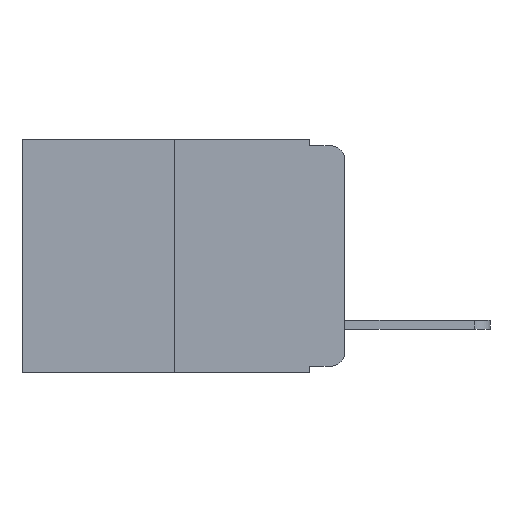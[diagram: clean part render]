
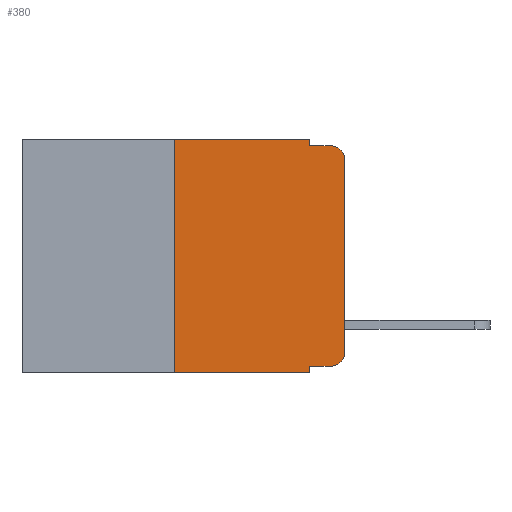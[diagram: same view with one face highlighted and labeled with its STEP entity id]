
A CAD part, left-side view. The second image highlights one B-rep face of the part: STEP entity #380.
In plain terms, the highlighted planar face has unit normal (-1, 0, 0).
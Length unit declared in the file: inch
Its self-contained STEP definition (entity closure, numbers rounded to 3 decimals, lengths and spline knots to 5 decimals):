
#11 = CARTESIAN_POINT ( 'NONE',  ( 0., 0.051, -0.333 ) ) ;
#145 = CARTESIAN_POINT ( 'NONE',  ( 0., 0., -0.03 ) ) ;
#380 = ADVANCED_FACE ( 'NONE', ( #26238 ), #19855, .F. ) ;
#389 = DIRECTION ( 'NONE',  ( 0., -1., 0. ) ) ;
#638 = VERTEX_POINT ( 'NONE', #8819 ) ;
#847 = DIRECTION ( 'NONE',  ( 0., 0., -1. ) ) ;
#1502 = LINE ( 'NONE', #21093, #23207 ) ;
#1549 = EDGE_CURVE ( 'NONE', #16674, #19604, #25883, .T. ) ;
#2672 = CARTESIAN_POINT ( 'NONE',  ( 0., 0.051, -0.333 ) ) ;
#2821 = DIRECTION ( 'NONE',  ( 1., 0., 0. ) ) ;
#3396 = ORIENTED_EDGE ( 'NONE', *, *, #11394, .F. ) ;
#3558 = VERTEX_POINT ( 'NONE', #25759 ) ;
#4065 = DIRECTION ( 'NONE',  ( 0., 0., -1. ) ) ;
#4387 = CARTESIAN_POINT ( 'NONE',  ( 0., 0.051, 0. ) ) ;
#4966 = ORIENTED_EDGE ( 'NONE', *, *, #20659, .F. ) ;
#5170 = VECTOR ( 'NONE', #23710, 39.37008 ) ;
#5179 = CARTESIAN_POINT ( 'NONE',  ( 0., 0.02, -0.03 ) ) ;
#5400 = CARTESIAN_POINT ( 'NONE',  ( 0., 0.051, -0.01 ) ) ;
#5989 = EDGE_CURVE ( 'NONE', #12069, #20249, #1502, .T. ) ;
#6025 = ORIENTED_EDGE ( 'NONE', *, *, #10478, .T. ) ;
#6357 = LINE ( 'NONE', #5400, #10859 ) ;
#6811 = VECTOR ( 'NONE', #18965, 39.37008 ) ;
#7145 = EDGE_CURVE ( 'NONE', #23434, #12368, #23987, .T. ) ;
#7279 = CARTESIAN_POINT ( 'NONE',  ( 0., 0.051, 0. ) ) ;
#7576 = VERTEX_POINT ( 'NONE', #20404 ) ;
#7579 = DIRECTION ( 'NONE',  ( 0., 0., -1. ) ) ;
#8819 = CARTESIAN_POINT ( 'NONE',  ( 0., 0., -0.313 ) ) ;
#8915 = ORIENTED_EDGE ( 'NONE', *, *, #20207, .T. ) ;
#9317 = ORIENTED_EDGE ( 'NONE', *, *, #16823, .F. ) ;
#9925 = CARTESIAN_POINT ( 'NONE',  ( 0., 0.473, 0. ) ) ;
#10348 = AXIS2_PLACEMENT_3D ( 'NONE', #23333, #2821, #18518 ) ;
#10478 = EDGE_CURVE ( 'NONE', #638, #13058, #14177, .T. ) ;
#10859 = VECTOR ( 'NONE', #23642, 39.37008 ) ;
#10998 = EDGE_LOOP ( 'NONE', ( #6025, #8915, #18679, #19288, #3396, #4966, #12213, #9317, #21693, #17779 ) ) ;
#11394 = EDGE_CURVE ( 'NONE', #3558, #16674, #15629, .T. ) ;
#12069 = VERTEX_POINT ( 'NONE', #15549 ) ;
#12213 = ORIENTED_EDGE ( 'NONE', *, *, #5989, .T. ) ;
#12259 = CARTESIAN_POINT ( 'NONE',  ( 0., 0., 0. ) ) ;
#12368 = VERTEX_POINT ( 'NONE', #16538 ) ;
#12529 = LINE ( 'NONE', #26191, #6811 ) ;
#13058 = VERTEX_POINT ( 'NONE', #145 ) ;
#14065 = CARTESIAN_POINT ( 'NONE',  ( 0., 0.051, 0. ) ) ;
#14177 = LINE ( 'NONE', #12259, #15356 ) ;
#14287 = DIRECTION ( 'NONE',  ( 0., 0., 1. ) ) ;
#14401 = DIRECTION ( 'NONE',  ( -1., 0., 0. ) ) ;
#14963 = EDGE_CURVE ( 'NONE', #19604, #7576, #6357, .T. ) ;
#15356 = VECTOR ( 'NONE', #14287, 39.37008 ) ;
#15549 = CARTESIAN_POINT ( 'NONE',  ( 0., 0.25, -0.343 ) ) ;
#15629 = LINE ( 'NONE', #9925, #20220 ) ;
#16182 = AXIS2_PLACEMENT_3D ( 'NONE', #25723, #14401, #847 ) ;
#16419 = LINE ( 'NONE', #14065, #5170 ) ;
#16538 = CARTESIAN_POINT ( 'NONE',  ( 0., 0.02, -0.333 ) ) ;
#16674 = VERTEX_POINT ( 'NONE', #7279 ) ;
#16823 = EDGE_CURVE ( 'NONE', #23434, #20249, #16419, .T. ) ;
#17143 = CIRCLE ( 'NONE', #16182, 0.02 ) ;
#17779 = ORIENTED_EDGE ( 'NONE', *, *, #23666, .T. ) ;
#17806 = CARTESIAN_POINT ( 'NONE',  ( 0., 0.051, -0.343 ) ) ;
#18518 = DIRECTION ( 'NONE',  ( 0., 0., -1. ) ) ;
#18679 = ORIENTED_EDGE ( 'NONE', *, *, #14963, .F. ) ;
#18965 = DIRECTION ( 'NONE',  ( 0., 0., 1. ) ) ;
#19009 = VECTOR ( 'NONE', #389, 39.37008 ) ;
#19288 = ORIENTED_EDGE ( 'NONE', *, *, #1549, .F. ) ;
#19308 = CIRCLE ( 'NONE', #20060, 0.02 ) ;
#19604 = VERTEX_POINT ( 'NONE', #24099 ) ;
#19671 = DIRECTION ( 'NONE',  ( -1., 0., 0. ) ) ;
#19855 = PLANE ( 'NONE',  #10348 ) ;
#20060 = AXIS2_PLACEMENT_3D ( 'NONE', #5179, #19671, #7579 ) ;
#20207 = EDGE_CURVE ( 'NONE', #13058, #7576, #19308, .T. ) ;
#20220 = VECTOR ( 'NONE', #25337, 39.37008 ) ;
#20249 = VERTEX_POINT ( 'NONE', #17806 ) ;
#20404 = CARTESIAN_POINT ( 'NONE',  ( 0., 0.02, -0.01 ) ) ;
#20659 = EDGE_CURVE ( 'NONE', #12069, #3558, #12529, .T. ) ;
#21059 = DIRECTION ( 'NONE',  ( 0., -1., 0. ) ) ;
#21093 = CARTESIAN_POINT ( 'NONE',  ( 0., 0.473, -0.343 ) ) ;
#21693 = ORIENTED_EDGE ( 'NONE', *, *, #7145, .T. ) ;
#23207 = VECTOR ( 'NONE', #21059, 39.37008 ) ;
#23333 = CARTESIAN_POINT ( 'NONE',  ( 0., 0.473, 0. ) ) ;
#23434 = VERTEX_POINT ( 'NONE', #2672 ) ;
#23642 = DIRECTION ( 'NONE',  ( 0., -1., 0. ) ) ;
#23666 = EDGE_CURVE ( 'NONE', #12368, #638, #17143, .T. ) ;
#23710 = DIRECTION ( 'NONE',  ( 0., 0., -1. ) ) ;
#23987 = LINE ( 'NONE', #11, #19009 ) ;
#24099 = CARTESIAN_POINT ( 'NONE',  ( 0., 0.051, -0.01 ) ) ;
#24729 = VECTOR ( 'NONE', #4065, 39.37008 ) ;
#25337 = DIRECTION ( 'NONE',  ( 0., -1., 0. ) ) ;
#25723 = CARTESIAN_POINT ( 'NONE',  ( 0., 0.02, -0.313 ) ) ;
#25759 = CARTESIAN_POINT ( 'NONE',  ( 0., 0.25, 0. ) ) ;
#25883 = LINE ( 'NONE', #4387, #24729 ) ;
#26191 = CARTESIAN_POINT ( 'NONE',  ( 0., 0.25, 0. ) ) ;
#26238 = FACE_OUTER_BOUND ( 'NONE', #10998, .T. ) ;
